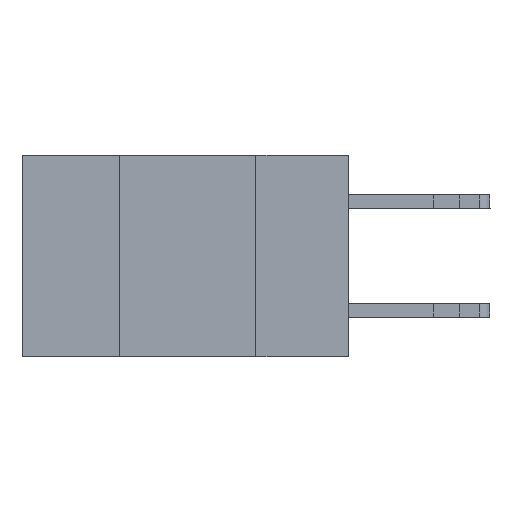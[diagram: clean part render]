
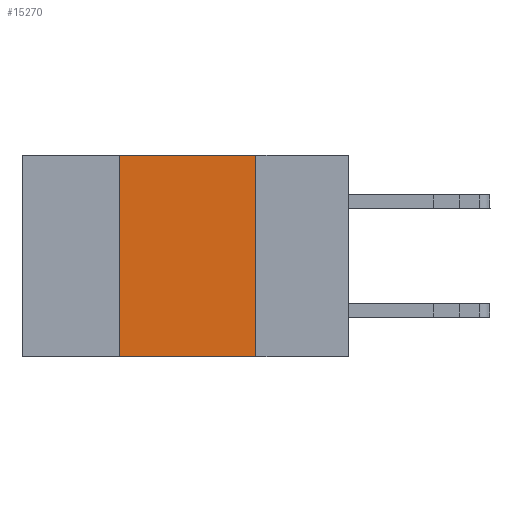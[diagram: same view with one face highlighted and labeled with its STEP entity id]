
A CAD part, left-side view. The second image highlights one B-rep face of the part: STEP entity #15270.
In plain terms, the highlighted planar face has unit normal (-1, 0, 0).
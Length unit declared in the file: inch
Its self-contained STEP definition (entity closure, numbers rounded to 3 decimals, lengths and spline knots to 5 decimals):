
#164 = CARTESIAN_POINT ( 'NONE',  ( 0., 0.17, 0. ) ) ;
#907 = CARTESIAN_POINT ( 'NONE',  ( 0., 0.17, -0.37 ) ) ;
#924 = VECTOR ( 'NONE', #12530, 39.37008 ) ;
#2255 = DIRECTION ( 'NONE',  ( 1., 0., 0. ) ) ;
#2477 = CARTESIAN_POINT ( 'NONE',  ( 0., 0.6, 0. ) ) ;
#3193 = VECTOR ( 'NONE', #6376, 39.37008 ) ;
#3869 = VECTOR ( 'NONE', #12195, 39.37008 ) ;
#3975 = VERTEX_POINT ( 'NONE', #164 ) ;
#4365 = DIRECTION ( 'NONE',  ( 0., 0., -1. ) ) ;
#5784 = ORIENTED_EDGE ( 'NONE', *, *, #20737, .T. ) ;
#5834 = LINE ( 'NONE', #17406, #924 ) ;
#6376 = DIRECTION ( 'NONE',  ( 0., -1., 0. ) ) ;
#6572 = ORIENTED_EDGE ( 'NONE', *, *, #8127, .F. ) ;
#7315 = CARTESIAN_POINT ( 'NONE',  ( 0., 0.42, -0.37 ) ) ;
#8036 = LINE ( 'NONE', #21611, #3193 ) ;
#8127 = EDGE_CURVE ( 'NONE', #17698, #13632, #5834, .T. ) ;
#9240 = DIRECTION ( 'NONE',  ( 0., 0., -1. ) ) ;
#9711 = EDGE_CURVE ( 'NONE', #13632, #3975, #8036, .T. ) ;
#11356 = VERTEX_POINT ( 'NONE', #17039 ) ;
#11922 = AXIS2_PLACEMENT_3D ( 'NONE', #2477, #2255, #9240 ) ;
#12123 = ORIENTED_EDGE ( 'NONE', *, *, #13607, .F. ) ;
#12195 = DIRECTION ( 'NONE',  ( 0., -1., 0. ) ) ;
#12530 = DIRECTION ( 'NONE',  ( 0., 0., 1. ) ) ;
#13607 = EDGE_CURVE ( 'NONE', #3975, #11356, #19366, .T. ) ;
#13632 = VERTEX_POINT ( 'NONE', #17484 ) ;
#13740 = LINE ( 'NONE', #20305, #3869 ) ;
#14155 = EDGE_LOOP ( 'NONE', ( #12123, #18185, #6572, #5784 ) ) ;
#15270 = ADVANCED_FACE ( 'NONE', ( #17691 ), #16151, .F. ) ;
#15325 = VECTOR ( 'NONE', #4365, 39.37008 ) ;
#16151 = PLANE ( 'NONE',  #11922 ) ;
#17039 = CARTESIAN_POINT ( 'NONE',  ( 0., 0.17, -0.37 ) ) ;
#17406 = CARTESIAN_POINT ( 'NONE',  ( 0., 0.42, -0.37 ) ) ;
#17484 = CARTESIAN_POINT ( 'NONE',  ( 0., 0.42, 0. ) ) ;
#17691 = FACE_OUTER_BOUND ( 'NONE', #14155, .T. ) ;
#17698 = VERTEX_POINT ( 'NONE', #7315 ) ;
#18185 = ORIENTED_EDGE ( 'NONE', *, *, #9711, .F. ) ;
#19366 = LINE ( 'NONE', #907, #15325 ) ;
#20305 = CARTESIAN_POINT ( 'NONE',  ( 0., 0.6, -0.37 ) ) ;
#20737 = EDGE_CURVE ( 'NONE', #17698, #11356, #13740, .T. ) ;
#21611 = CARTESIAN_POINT ( 'NONE',  ( 0., 0.6, 0. ) ) ;
